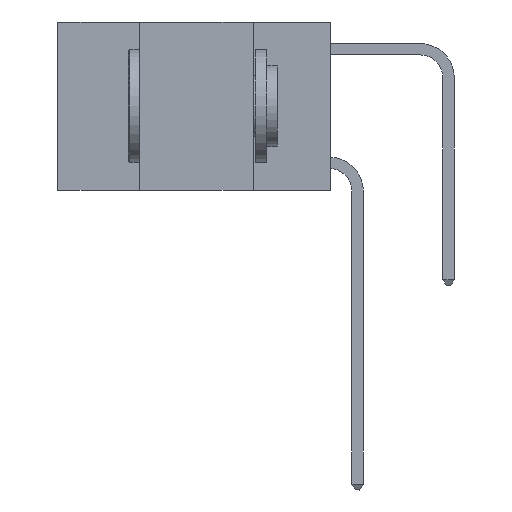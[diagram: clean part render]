
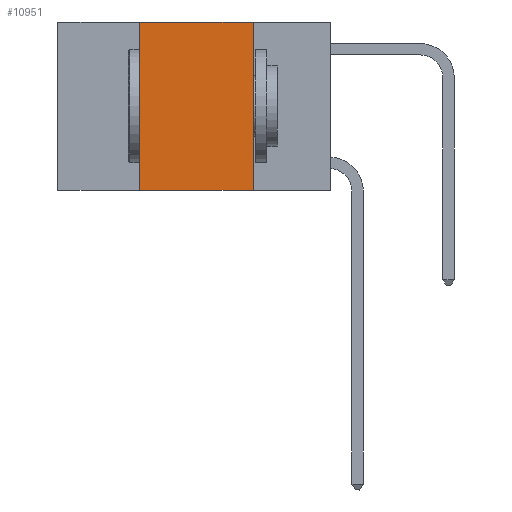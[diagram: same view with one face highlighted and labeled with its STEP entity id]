
A CAD part, left-side view. The second image highlights one B-rep face of the part: STEP entity #10951.
In plain terms, the highlighted planar face has unit normal (-1, 0, 0).
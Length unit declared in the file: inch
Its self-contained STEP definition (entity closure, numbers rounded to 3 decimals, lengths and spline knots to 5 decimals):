
#500 = VECTOR ( 'NONE', #3311, 39.37008 ) ;
#975 = LINE ( 'NONE', #2093, #500 ) ;
#1246 = LINE ( 'NONE', #6940, #4474 ) ;
#1489 = CARTESIAN_POINT ( 'NONE',  ( 0., 0.6, 0. ) ) ;
#1540 = CARTESIAN_POINT ( 'NONE',  ( 0., 0.6, 0. ) ) ;
#2093 = CARTESIAN_POINT ( 'NONE',  ( 0., 0.42, 0. ) ) ;
#2281 = VERTEX_POINT ( 'NONE', #15487 ) ;
#2351 = EDGE_CURVE ( 'NONE', #8437, #14944, #9143, .T. ) ;
#3103 = LINE ( 'NONE', #7617, #3554 ) ;
#3311 = DIRECTION ( 'NONE',  ( 0., 0., 1. ) ) ;
#3486 = EDGE_CURVE ( 'NONE', #14944, #2281, #1246, .T. ) ;
#3554 = VECTOR ( 'NONE', #13384, 39.37008 ) ;
#4441 = DIRECTION ( 'NONE',  ( 0., -1., 0. ) ) ;
#4474 = VECTOR ( 'NONE', #15858, 39.37008 ) ;
#6940 = CARTESIAN_POINT ( 'NONE',  ( 0., 0.17, 0. ) ) ;
#7381 = CARTESIAN_POINT ( 'NONE',  ( 0., 0.42, -0.37 ) ) ;
#7617 = CARTESIAN_POINT ( 'NONE',  ( 0., 0.6, -0.37 ) ) ;
#7694 = CARTESIAN_POINT ( 'NONE',  ( 0., 0.42, 0. ) ) ;
#8113 = FACE_OUTER_BOUND ( 'NONE', #15204, .T. ) ;
#8239 = ORIENTED_EDGE ( 'NONE', *, *, #2351, .F. ) ;
#8437 = VERTEX_POINT ( 'NONE', #7694 ) ;
#8728 = DIRECTION ( 'NONE',  ( 1., 0., 0. ) ) ;
#9143 = LINE ( 'NONE', #1540, #13740 ) ;
#10251 = VERTEX_POINT ( 'NONE', #7381 ) ;
#10478 = EDGE_CURVE ( 'NONE', #10251, #8437, #975, .T. ) ;
#10951 = ADVANCED_FACE ( 'NONE', ( #8113 ), #16072, .F. ) ;
#12910 = ORIENTED_EDGE ( 'NONE', *, *, #3486, .F. ) ;
#13171 = DIRECTION ( 'NONE',  ( 0., 0., -1. ) ) ;
#13384 = DIRECTION ( 'NONE',  ( 0., -1., 0. ) ) ;
#13740 = VECTOR ( 'NONE', #4441, 39.37008 ) ;
#14034 = ORIENTED_EDGE ( 'NONE', *, *, #10478, .F. ) ;
#14784 = CARTESIAN_POINT ( 'NONE',  ( 0., 0.17, 0. ) ) ;
#14944 = VERTEX_POINT ( 'NONE', #14784 ) ;
#15204 = EDGE_LOOP ( 'NONE', ( #12910, #8239, #14034, #15338 ) ) ;
#15338 = ORIENTED_EDGE ( 'NONE', *, *, #17001, .T. ) ;
#15487 = CARTESIAN_POINT ( 'NONE',  ( 0., 0.17, -0.37 ) ) ;
#15858 = DIRECTION ( 'NONE',  ( 0., 0., -1. ) ) ;
#16072 = PLANE ( 'NONE',  #16117 ) ;
#16117 = AXIS2_PLACEMENT_3D ( 'NONE', #1489, #8728, #13171 ) ;
#17001 = EDGE_CURVE ( 'NONE', #10251, #2281, #3103, .T. ) ;
